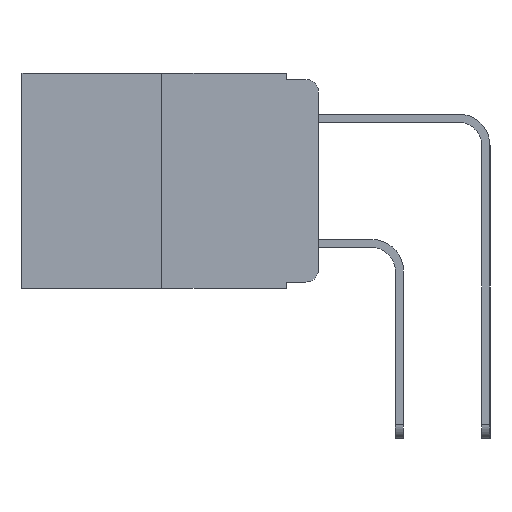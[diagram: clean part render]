
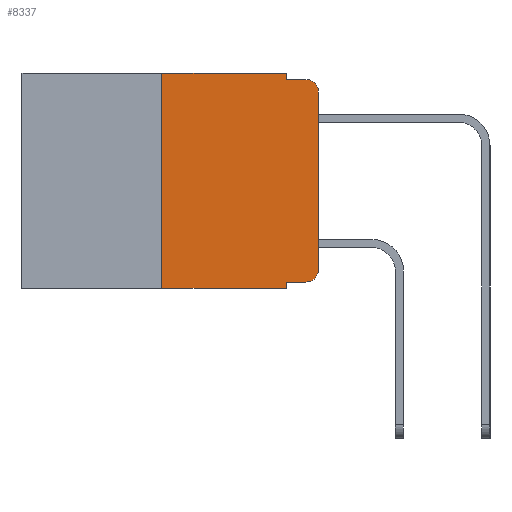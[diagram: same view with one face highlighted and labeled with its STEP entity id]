
A CAD part, left-side view. The second image highlights one B-rep face of the part: STEP entity #8337.
In plain terms, the highlighted planar face has unit normal (-1, 0, 0).
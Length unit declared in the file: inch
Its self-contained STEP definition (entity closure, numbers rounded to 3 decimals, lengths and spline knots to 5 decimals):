
#313 = ORIENTED_EDGE ( 'NONE', *, *, #11449, .F. ) ;
#432 = AXIS2_PLACEMENT_3D ( 'NONE', #6841, #17249, #8472 ) ;
#1601 = FACE_OUTER_BOUND ( 'NONE', #17730, .T. ) ;
#2016 = VERTEX_POINT ( 'NONE', #14291 ) ;
#2145 = ORIENTED_EDGE ( 'NONE', *, *, #7046, .T. ) ;
#2250 = VERTEX_POINT ( 'NONE', #11990 ) ;
#2753 = VECTOR ( 'NONE', #3220, 39.37008 ) ;
#2864 = PLANE ( 'NONE',  #16421 ) ;
#2891 = LINE ( 'NONE', #10801, #17651 ) ;
#3059 = CARTESIAN_POINT ( 'NONE',  ( 0., 0.051, -0.333 ) ) ;
#3220 = DIRECTION ( 'NONE',  ( 0., -1., 0. ) ) ;
#3350 = ORIENTED_EDGE ( 'NONE', *, *, #14360, .F. ) ;
#4214 = CARTESIAN_POINT ( 'NONE',  ( 0., 0.25, 0. ) ) ;
#4244 = VERTEX_POINT ( 'NONE', #14269 ) ;
#4247 = LINE ( 'NONE', #13748, #12474 ) ;
#4347 = AXIS2_PLACEMENT_3D ( 'NONE', #15245, #6279, #16710 ) ;
#4517 = DIRECTION ( 'NONE',  ( 0., 0., -1. ) ) ;
#4898 = CARTESIAN_POINT ( 'NONE',  ( 0., 0.473, 0. ) ) ;
#5305 = LINE ( 'NONE', #7866, #9549 ) ;
#5396 = VERTEX_POINT ( 'NONE', #9335 ) ;
#5873 = DIRECTION ( 'NONE',  ( 0., 0., 1. ) ) ;
#6184 = ORIENTED_EDGE ( 'NONE', *, *, #16444, .F. ) ;
#6279 = DIRECTION ( 'NONE',  ( -1., 0., 0. ) ) ;
#6644 = VERTEX_POINT ( 'NONE', #18325 ) ;
#6708 = ORIENTED_EDGE ( 'NONE', *, *, #14595, .T. ) ;
#6841 = CARTESIAN_POINT ( 'NONE',  ( 0., 0.02, -0.03 ) ) ;
#7046 = EDGE_CURVE ( 'NONE', #2016, #2250, #11978, .T. ) ;
#7073 = VECTOR ( 'NONE', #14663, 39.37008 ) ;
#7113 = CIRCLE ( 'NONE', #432, 0.02 ) ;
#7369 = EDGE_CURVE ( 'NONE', #11149, #18358, #2891, .T. ) ;
#7381 = CARTESIAN_POINT ( 'NONE',  ( 0., 0.051, -0.333 ) ) ;
#7448 = ORIENTED_EDGE ( 'NONE', *, *, #16306, .F. ) ;
#7576 = LINE ( 'NONE', #14609, #7073 ) ;
#7866 = CARTESIAN_POINT ( 'NONE',  ( 0., 0.051, 0. ) ) ;
#7999 = VECTOR ( 'NONE', #16646, 39.37008 ) ;
#8337 = ADVANCED_FACE ( 'NONE', ( #1601 ), #2864, .F. ) ;
#8472 = DIRECTION ( 'NONE',  ( 0., 0., -1. ) ) ;
#8691 = VERTEX_POINT ( 'NONE', #11356 ) ;
#9195 = CARTESIAN_POINT ( 'NONE',  ( 0., 0., -0.03 ) ) ;
#9251 = VERTEX_POINT ( 'NONE', #3059 ) ;
#9335 = CARTESIAN_POINT ( 'NONE',  ( 0., 0.051, 0. ) ) ;
#9372 = DIRECTION ( 'NONE',  ( 0., 0., -1. ) ) ;
#9421 = CARTESIAN_POINT ( 'NONE',  ( 0., 0.473, -0.343 ) ) ;
#9491 = EDGE_CURVE ( 'NONE', #18358, #11494, #7113, .T. ) ;
#9549 = VECTOR ( 'NONE', #16675, 39.37008 ) ;
#9902 = ORIENTED_EDGE ( 'NONE', *, *, #18247, .T. ) ;
#10334 = ORIENTED_EDGE ( 'NONE', *, *, #9491, .T. ) ;
#10478 = EDGE_CURVE ( 'NONE', #4244, #11494, #7576, .T. ) ;
#10801 = CARTESIAN_POINT ( 'NONE',  ( 0., 0., 0. ) ) ;
#11149 = VERTEX_POINT ( 'NONE', #11746 ) ;
#11356 = CARTESIAN_POINT ( 'NONE',  ( 0., 0.25, 0. ) ) ;
#11449 = EDGE_CURVE ( 'NONE', #5396, #4244, #4247, .T. ) ;
#11494 = VERTEX_POINT ( 'NONE', #19629 ) ;
#11746 = CARTESIAN_POINT ( 'NONE',  ( 0., 0., -0.313 ) ) ;
#11978 = LINE ( 'NONE', #9421, #7999 ) ;
#11990 = CARTESIAN_POINT ( 'NONE',  ( 0., 0.051, -0.343 ) ) ;
#12474 = VECTOR ( 'NONE', #9372, 39.37008 ) ;
#12885 = VECTOR ( 'NONE', #13410, 39.37008 ) ;
#13345 = LINE ( 'NONE', #7381, #12885 ) ;
#13410 = DIRECTION ( 'NONE',  ( 0., -1., 0. ) ) ;
#13623 = CARTESIAN_POINT ( 'NONE',  ( 0., 0.473, 0. ) ) ;
#13679 = DIRECTION ( 'NONE',  ( 1., 0., 0. ) ) ;
#13748 = CARTESIAN_POINT ( 'NONE',  ( 0., 0.051, 0. ) ) ;
#14269 = CARTESIAN_POINT ( 'NONE',  ( 0., 0.051, -0.01 ) ) ;
#14291 = CARTESIAN_POINT ( 'NONE',  ( 0., 0.25, -0.343 ) ) ;
#14360 = EDGE_CURVE ( 'NONE', #2016, #8691, #15502, .T. ) ;
#14595 = EDGE_CURVE ( 'NONE', #6644, #11149, #19566, .T. ) ;
#14609 = CARTESIAN_POINT ( 'NONE',  ( 0., 0.051, -0.01 ) ) ;
#14663 = DIRECTION ( 'NONE',  ( 0., -1., 0. ) ) ;
#14973 = LINE ( 'NONE', #4898, #2753 ) ;
#15165 = DIRECTION ( 'NONE',  ( 0., 0., 1. ) ) ;
#15245 = CARTESIAN_POINT ( 'NONE',  ( 0., 0.02, -0.313 ) ) ;
#15502 = LINE ( 'NONE', #4214, #18921 ) ;
#16306 = EDGE_CURVE ( 'NONE', #9251, #2250, #5305, .T. ) ;
#16421 = AXIS2_PLACEMENT_3D ( 'NONE', #13623, #13679, #4517 ) ;
#16444 = EDGE_CURVE ( 'NONE', #8691, #5396, #14973, .T. ) ;
#16646 = DIRECTION ( 'NONE',  ( 0., -1., 0. ) ) ;
#16675 = DIRECTION ( 'NONE',  ( 0., 0., -1. ) ) ;
#16710 = DIRECTION ( 'NONE',  ( 0., 0., -1. ) ) ;
#17249 = DIRECTION ( 'NONE',  ( -1., 0., 0. ) ) ;
#17651 = VECTOR ( 'NONE', #15165, 39.37008 ) ;
#17730 = EDGE_LOOP ( 'NONE', ( #18716, #10334, #19622, #313, #6184, #3350, #2145, #7448, #9902, #6708 ) ) ;
#18247 = EDGE_CURVE ( 'NONE', #9251, #6644, #13345, .T. ) ;
#18325 = CARTESIAN_POINT ( 'NONE',  ( 0., 0.02, -0.333 ) ) ;
#18358 = VERTEX_POINT ( 'NONE', #9195 ) ;
#18716 = ORIENTED_EDGE ( 'NONE', *, *, #7369, .T. ) ;
#18921 = VECTOR ( 'NONE', #5873, 39.37008 ) ;
#19566 = CIRCLE ( 'NONE', #4347, 0.02 ) ;
#19622 = ORIENTED_EDGE ( 'NONE', *, *, #10478, .F. ) ;
#19629 = CARTESIAN_POINT ( 'NONE',  ( 0., 0.02, -0.01 ) ) ;
